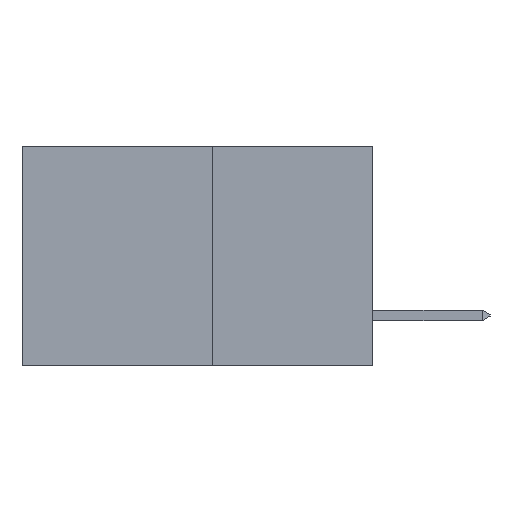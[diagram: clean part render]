
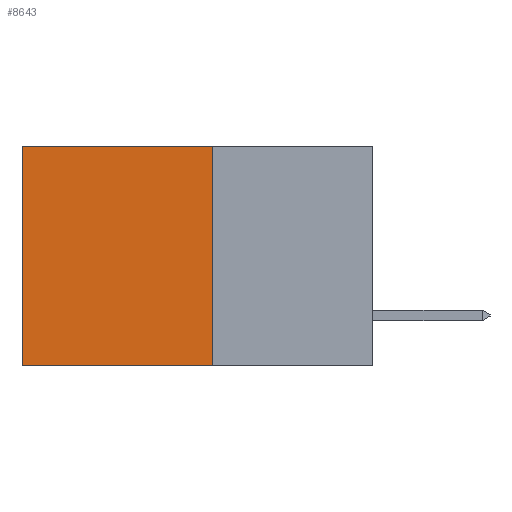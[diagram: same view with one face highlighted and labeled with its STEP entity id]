
A CAD part, left-side view. The second image highlights one B-rep face of the part: STEP entity #8643.
In plain terms, the highlighted planar face has unit normal (-1, 0, 0).
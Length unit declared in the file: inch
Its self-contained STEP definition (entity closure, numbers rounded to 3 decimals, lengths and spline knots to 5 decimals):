
#924 = VECTOR ( 'NONE', #9749, 39.37008 ) ;
#1568 = DIRECTION ( 'NONE',  ( 0., 1., 0. ) ) ;
#2030 = CARTESIAN_POINT ( 'NONE',  ( 0.277, 0.27, -0.37 ) ) ;
#2723 = CARTESIAN_POINT ( 'NONE',  ( 0.277, 0.27, -0.37 ) ) ;
#3269 = CARTESIAN_POINT ( 'NONE',  ( 0.277, 0.59, -0.37 ) ) ;
#3555 = LINE ( 'NONE', #3269, #6411 ) ;
#4264 = DIRECTION ( 'NONE',  ( 0., 0., -1. ) ) ;
#4690 = CARTESIAN_POINT ( 'NONE',  ( 0.277, 0.59, -0.37 ) ) ;
#4863 = EDGE_CURVE ( 'NONE', #5229, #5152, #6199, .T. ) ;
#5152 = VERTEX_POINT ( 'NONE', #6734 ) ;
#5229 = VERTEX_POINT ( 'NONE', #8247 ) ;
#5694 = VERTEX_POINT ( 'NONE', #4690 ) ;
#5808 = CARTESIAN_POINT ( 'NONE',  ( 0.277, 0.27, -0.37 ) ) ;
#5976 = AXIS2_PLACEMENT_3D ( 'NONE', #5808, #12044, #6752 ) ;
#6157 = ORIENTED_EDGE ( 'NONE', *, *, #11500, .F. ) ;
#6199 = LINE ( 'NONE', #9297, #924 ) ;
#6411 = VECTOR ( 'NONE', #4264, 39.37008 ) ;
#6429 = ORIENTED_EDGE ( 'NONE', *, *, #11107, .T. ) ;
#6457 = CARTESIAN_POINT ( 'NONE',  ( 0.277, 0.27, -0.37 ) ) ;
#6708 = VECTOR ( 'NONE', #7532, 39.37008 ) ;
#6734 = CARTESIAN_POINT ( 'NONE',  ( 0.277, 0.59, 0. ) ) ;
#6752 = DIRECTION ( 'NONE',  ( 0., 0., -1. ) ) ;
#7031 = VERTEX_POINT ( 'NONE', #2030 ) ;
#7313 = EDGE_LOOP ( 'NONE', ( #6429, #10898, #6157, #8548 ) ) ;
#7532 = DIRECTION ( 'NONE',  ( 0., 0., -1. ) ) ;
#8247 = CARTESIAN_POINT ( 'NONE',  ( 0.277, 0.27, 0. ) ) ;
#8262 = VECTOR ( 'NONE', #1568, 39.37008 ) ;
#8548 = ORIENTED_EDGE ( 'NONE', *, *, #4863, .T. ) ;
#8643 = ADVANCED_FACE ( 'NONE', ( #10507 ), #10266, .F. ) ;
#9077 = LINE ( 'NONE', #2723, #6708 ) ;
#9297 = CARTESIAN_POINT ( 'NONE',  ( 0.277, 0.27, 0. ) ) ;
#9749 = DIRECTION ( 'NONE',  ( 0., 1., 0. ) ) ;
#10266 = PLANE ( 'NONE',  #5976 ) ;
#10507 = FACE_OUTER_BOUND ( 'NONE', #7313, .T. ) ;
#10602 = LINE ( 'NONE', #6457, #8262 ) ;
#10719 = EDGE_CURVE ( 'NONE', #7031, #5694, #10602, .T. ) ;
#10898 = ORIENTED_EDGE ( 'NONE', *, *, #10719, .F. ) ;
#11107 = EDGE_CURVE ( 'NONE', #5152, #5694, #3555, .T. ) ;
#11500 = EDGE_CURVE ( 'NONE', #5229, #7031, #9077, .T. ) ;
#12044 = DIRECTION ( 'NONE',  ( 1., 0., 0. ) ) ;
